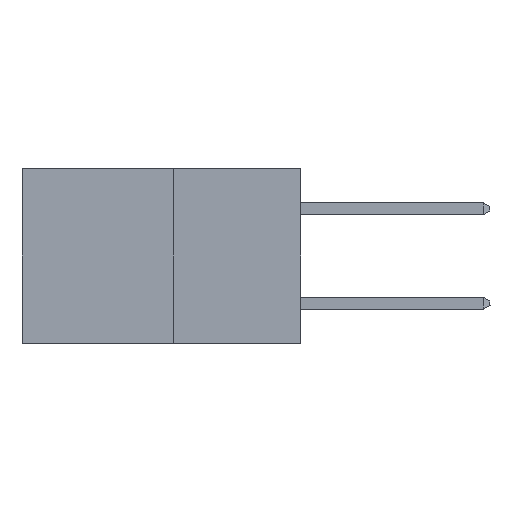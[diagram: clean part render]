
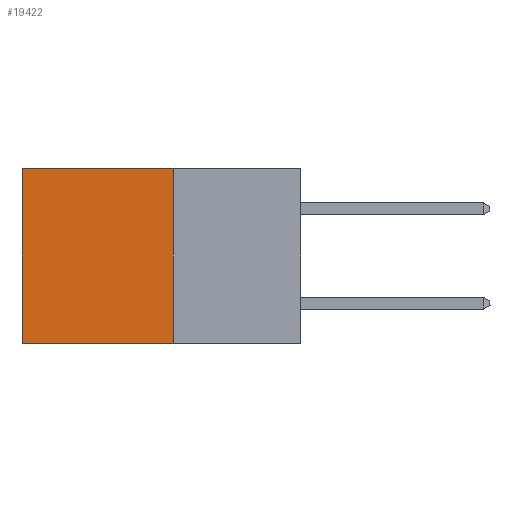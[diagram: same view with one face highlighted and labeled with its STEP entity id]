
A CAD part, left-side view. The second image highlights one B-rep face of the part: STEP entity #19422.
In plain terms, the highlighted planar face has unit normal (-1, 0, 0).
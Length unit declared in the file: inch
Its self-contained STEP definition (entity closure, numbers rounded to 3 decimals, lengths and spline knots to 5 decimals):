
#137 = CARTESIAN_POINT ( 'NONE',  ( 0.277, 0.27, -0.37 ) ) ;
#218 = FACE_OUTER_BOUND ( 'NONE', #1918, .T. ) ;
#828 = VECTOR ( 'NONE', #16037, 39.37008 ) ;
#959 = CARTESIAN_POINT ( 'NONE',  ( 0.277, 0.27, -0.37 ) ) ;
#1247 = EDGE_CURVE ( 'NONE', #4545, #16182, #9358, .T. ) ;
#1261 = PLANE ( 'NONE',  #9285 ) ;
#1918 = EDGE_LOOP ( 'NONE', ( #15551, #19955, #6706, #6846 ) ) ;
#3006 = DIRECTION ( 'NONE',  ( 0., 0., -1. ) ) ;
#3610 = VECTOR ( 'NONE', #20225, 39.37008 ) ;
#4545 = VERTEX_POINT ( 'NONE', #9308 ) ;
#5340 = LINE ( 'NONE', #9432, #828 ) ;
#6706 = ORIENTED_EDGE ( 'NONE', *, *, #9997, .F. ) ;
#6846 = ORIENTED_EDGE ( 'NONE', *, *, #1247, .T. ) ;
#7507 = LINE ( 'NONE', #17017, #3610 ) ;
#9277 = EDGE_CURVE ( 'NONE', #20199, #11193, #14546, .T. ) ;
#9285 = AXIS2_PLACEMENT_3D ( 'NONE', #19491, #13060, #3006 ) ;
#9308 = CARTESIAN_POINT ( 'NONE',  ( 0.277, 0.27, 0. ) ) ;
#9358 = LINE ( 'NONE', #9690, #17115 ) ;
#9432 = CARTESIAN_POINT ( 'NONE',  ( 0.277, 0.27, -0.37 ) ) ;
#9690 = CARTESIAN_POINT ( 'NONE',  ( 0.277, 0.27, 0. ) ) ;
#9997 = EDGE_CURVE ( 'NONE', #4545, #20199, #5340, .T. ) ;
#10118 = VECTOR ( 'NONE', #11142, 39.37008 ) ;
#11007 = DIRECTION ( 'NONE',  ( 0., 1., 0. ) ) ;
#11142 = DIRECTION ( 'NONE',  ( 0., 1., 0. ) ) ;
#11193 = VERTEX_POINT ( 'NONE', #15046 ) ;
#13060 = DIRECTION ( 'NONE',  ( 1., 0., 0. ) ) ;
#14546 = LINE ( 'NONE', #959, #10118 ) ;
#15046 = CARTESIAN_POINT ( 'NONE',  ( 0.277, 0.59, -0.37 ) ) ;
#15551 = ORIENTED_EDGE ( 'NONE', *, *, #20803, .T. ) ;
#16037 = DIRECTION ( 'NONE',  ( 0., 0., -1. ) ) ;
#16182 = VERTEX_POINT ( 'NONE', #18420 ) ;
#17017 = CARTESIAN_POINT ( 'NONE',  ( 0.277, 0.59, -0.37 ) ) ;
#17115 = VECTOR ( 'NONE', #11007, 39.37008 ) ;
#18420 = CARTESIAN_POINT ( 'NONE',  ( 0.277, 0.59, 0. ) ) ;
#19422 = ADVANCED_FACE ( 'NONE', ( #218 ), #1261, .F. ) ;
#19491 = CARTESIAN_POINT ( 'NONE',  ( 0.277, 0.27, -0.37 ) ) ;
#19955 = ORIENTED_EDGE ( 'NONE', *, *, #9277, .F. ) ;
#20199 = VERTEX_POINT ( 'NONE', #137 ) ;
#20225 = DIRECTION ( 'NONE',  ( 0., 0., -1. ) ) ;
#20803 = EDGE_CURVE ( 'NONE', #16182, #11193, #7507, .T. ) ;
